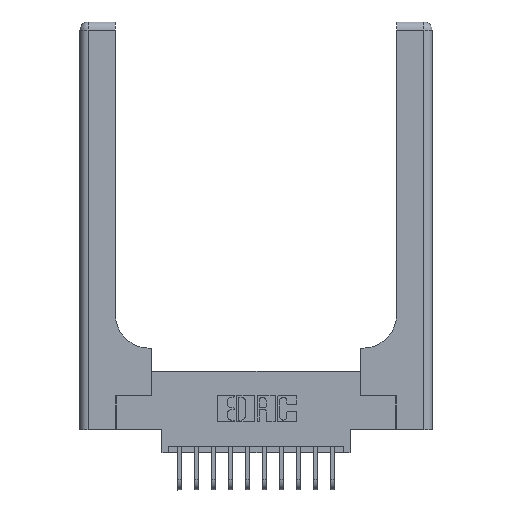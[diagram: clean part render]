
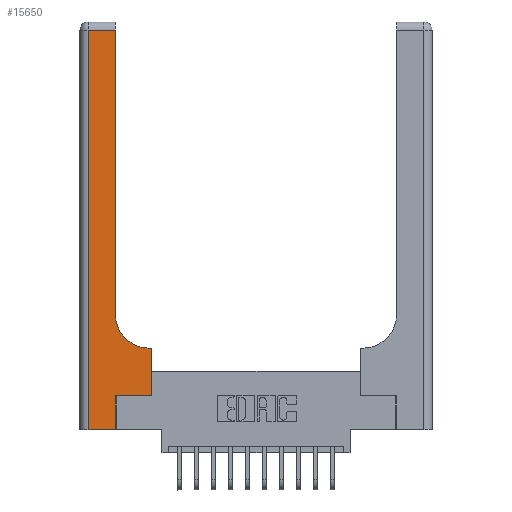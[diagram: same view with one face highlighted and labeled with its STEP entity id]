
A CAD part, top view. The second image highlights one B-rep face of the part: STEP entity #15650.
In plain terms, the highlighted planar face has unit normal (0, 0, 1).
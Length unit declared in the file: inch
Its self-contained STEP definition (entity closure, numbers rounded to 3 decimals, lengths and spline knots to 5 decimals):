
#110 = VERTEX_POINT ( 'NONE', #10188 ) ;
#166 = DIRECTION ( 'NONE',  ( 0., 1., 0. ) ) ;
#488 = EDGE_CURVE ( 'NONE', #9419, #8494, #10857, .T. ) ;
#542 = VERTEX_POINT ( 'NONE', #3402 ) ;
#621 = CARTESIAN_POINT ( 'NONE',  ( 0.06, 3., 0.37 ) ) ;
#973 = CARTESIAN_POINT ( 'NONE',  ( 0.26, 0.6, 0.37 ) ) ;
#1819 = ORIENTED_EDGE ( 'NONE', *, *, #9282, .T. ) ;
#1911 = CARTESIAN_POINT ( 'NONE',  ( 0.528, 0.6, 0.37 ) ) ;
#1966 = VERTEX_POINT ( 'NONE', #2817 ) ;
#2363 = DIRECTION ( 'NONE',  ( -1., 0., 0. ) ) ;
#2452 = CARTESIAN_POINT ( 'NONE',  ( 0.51, 0.85, 0.37 ) ) ;
#2714 = VERTEX_POINT ( 'NONE', #6482 ) ;
#2807 = DIRECTION ( 'NONE',  ( 1., 0., 0. ) ) ;
#2817 = CARTESIAN_POINT ( 'NONE',  ( 0.26, 0.85, 0.37 ) ) ;
#3070 = CARTESIAN_POINT ( 'NONE',  ( 0.528, 0.25, 0.37 ) ) ;
#3091 = DIRECTION ( 'NONE',  ( 0., -1., 0. ) ) ;
#3169 = LINE ( 'NONE', #621, #8544 ) ;
#3264 = DIRECTION ( 'NONE',  ( -1., 0., 0. ) ) ;
#3323 = VECTOR ( 'NONE', #11056, 39.37008 ) ;
#3402 = CARTESIAN_POINT ( 'NONE',  ( 0.26, 2.94, 0.37 ) ) ;
#3530 = CARTESIAN_POINT ( 'NONE',  ( 0.265, 0., 0.37 ) ) ;
#3709 = LINE ( 'NONE', #3962, #15312 ) ;
#3835 = LINE ( 'NONE', #15267, #15212 ) ;
#3854 = DIRECTION ( 'NONE',  ( 1., 0., 0. ) ) ;
#3962 = CARTESIAN_POINT ( 'NONE',  ( 0.26, 3., 0.37 ) ) ;
#4029 = EDGE_LOOP ( 'NONE', ( #16174, #8709, #1819, #15209, #11479, #6143, #4430, #15805, #7879 ) ) ;
#4043 = EDGE_CURVE ( 'NONE', #1966, #542, #3709, .T. ) ;
#4430 = ORIENTED_EDGE ( 'NONE', *, *, #488, .T. ) ;
#4512 = CARTESIAN_POINT ( 'NONE',  ( 0., 2.94, 0.37 ) ) ;
#4552 = CARTESIAN_POINT ( 'NONE',  ( 0.06, 0., 0.37 ) ) ;
#4678 = CARTESIAN_POINT ( 'NONE',  ( 0.265, 0.25, 0.37 ) ) ;
#4904 = CARTESIAN_POINT ( 'NONE',  ( 0.528, 0.25, 0.37 ) ) ;
#5142 = VECTOR ( 'NONE', #2807, 39.37008 ) ;
#5425 = VERTEX_POINT ( 'NONE', #3530 ) ;
#5824 = CARTESIAN_POINT ( 'NONE',  ( 0.51, 0.6, 0.37 ) ) ;
#5956 = EDGE_CURVE ( 'NONE', #5425, #2714, #3835, .T. ) ;
#6143 = ORIENTED_EDGE ( 'NONE', *, *, #11870, .T. ) ;
#6482 = CARTESIAN_POINT ( 'NONE',  ( 0.265, 0.25, 0.37 ) ) ;
#6677 = VERTEX_POINT ( 'NONE', #4552 ) ;
#6786 = FACE_OUTER_BOUND ( 'NONE', #4029, .T. ) ;
#7269 = DIRECTION ( 'NONE',  ( 0., 0., -1. ) ) ;
#7879 = ORIENTED_EDGE ( 'NONE', *, *, #16207, .T. ) ;
#7965 = PLANE ( 'NONE',  #14787 ) ;
#8043 = DIRECTION ( 'NONE',  ( -1., 0., 0. ) ) ;
#8391 = CIRCLE ( 'NONE', #15527, 0.25 ) ;
#8494 = VERTEX_POINT ( 'NONE', #1911 ) ;
#8544 = VECTOR ( 'NONE', #3091, 39.37008 ) ;
#8709 = ORIENTED_EDGE ( 'NONE', *, *, #12850, .T. ) ;
#9282 = EDGE_CURVE ( 'NONE', #110, #6677, #3169, .T. ) ;
#9419 = VERTEX_POINT ( 'NONE', #4904 ) ;
#10188 = CARTESIAN_POINT ( 'NONE',  ( 0.06, 2.94, 0.37 ) ) ;
#10857 = LINE ( 'NONE', #3070, #13017 ) ;
#11056 = DIRECTION ( 'NONE',  ( 1., 0., 0. ) ) ;
#11215 = EDGE_CURVE ( 'NONE', #6677, #5425, #11491, .T. ) ;
#11479 = ORIENTED_EDGE ( 'NONE', *, *, #5956, .T. ) ;
#11491 = LINE ( 'NONE', #14153, #5142 ) ;
#11870 = EDGE_CURVE ( 'NONE', #2714, #9419, #12217, .T. ) ;
#12131 = LINE ( 'NONE', #973, #12598 ) ;
#12217 = LINE ( 'NONE', #4678, #3323 ) ;
#12323 = VECTOR ( 'NONE', #3264, 39.37008 ) ;
#12598 = VECTOR ( 'NONE', #2363, 39.37008 ) ;
#12850 = EDGE_CURVE ( 'NONE', #542, #110, #14616, .T. ) ;
#13017 = VECTOR ( 'NONE', #13260, 39.37008 ) ;
#13021 = CARTESIAN_POINT ( 'NONE',  ( 0., 3., 0.37 ) ) ;
#13029 = EDGE_CURVE ( 'NONE', #8494, #13034, #12131, .T. ) ;
#13034 = VERTEX_POINT ( 'NONE', #5824 ) ;
#13260 = DIRECTION ( 'NONE',  ( 0., 1., 0. ) ) ;
#13702 = DIRECTION ( 'NONE',  ( 0., 1., 0. ) ) ;
#13719 = DIRECTION ( 'NONE',  ( 0., 0., -1. ) ) ;
#14153 = CARTESIAN_POINT ( 'NONE',  ( 0., 0., 0.37 ) ) ;
#14616 = LINE ( 'NONE', #4512, #12323 ) ;
#14787 = AXIS2_PLACEMENT_3D ( 'NONE', #13021, #7269, #8043 ) ;
#15209 = ORIENTED_EDGE ( 'NONE', *, *, #11215, .T. ) ;
#15212 = VECTOR ( 'NONE', #13702, 39.37008 ) ;
#15267 = CARTESIAN_POINT ( 'NONE',  ( 0.265, 0., 0.37 ) ) ;
#15312 = VECTOR ( 'NONE', #166, 39.37008 ) ;
#15527 = AXIS2_PLACEMENT_3D ( 'NONE', #2452, #13719, #3854 ) ;
#15650 = ADVANCED_FACE ( 'NONE', ( #6786 ), #7965, .F. ) ;
#15805 = ORIENTED_EDGE ( 'NONE', *, *, #13029, .T. ) ;
#16174 = ORIENTED_EDGE ( 'NONE', *, *, #4043, .T. ) ;
#16207 = EDGE_CURVE ( 'NONE', #13034, #1966, #8391, .T. ) ;
